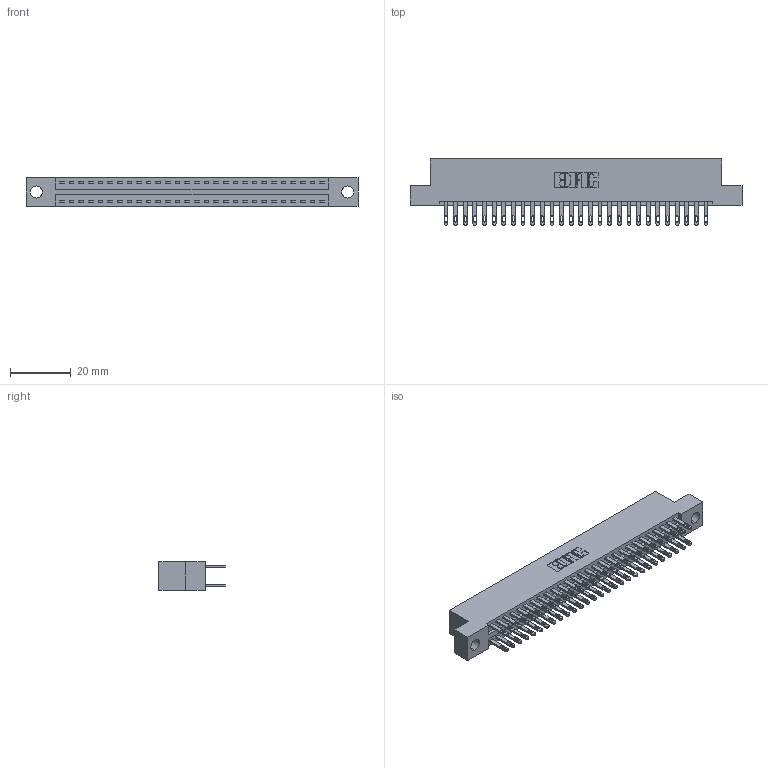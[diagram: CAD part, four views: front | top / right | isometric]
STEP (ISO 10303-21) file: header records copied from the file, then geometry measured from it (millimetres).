
FILE_DESCRIPTION (( 'STEP AP203' ), '1' );
FILE_NAME ('346-056-500-204.STEP', '2022-05-21T04:47:54', ( '' ), ( '' ), 'SwSTEP 2.0', 'SolidWorks 2020', '' );
FILE_SCHEMA (( 'CONFIG_CONTROL_DESIGN' ));
Length unit declared in the file: inch
Products named in the file (3): 346-056-500-204; 346 Part_Flush Mounting Lugs - 0.156 Dia-TH; 345-292-001_345-293-100
Assembly tree (57 placements, depth 2):
  346-056-500-204
    346 Part_Flush Mounting Lugs - 0.156 Dia-TH
    345-292-001_345-293-100  x56
Bounding box: 109.47 x 21.84 x 9.4 mm (x, y, z)
Volume: 10631.5 mm3; surface area: 14827.7 mm2
Topology: 57 solids, 57 shells, 2824 faces, 8597 edges, 5730 vertices
Faces by surface type: plane 1714, cylinder 1110
Entity records: 20507 total; most frequent: CARTESIAN_POINT 3402, ORIENTED_EDGE 3334, DIRECTION 3051, EDGE_CURVE 1667, LINE 1419, VECTOR 1419, VERTEX_POINT 1110, AXIS2_PLACEMENT_3D 816
